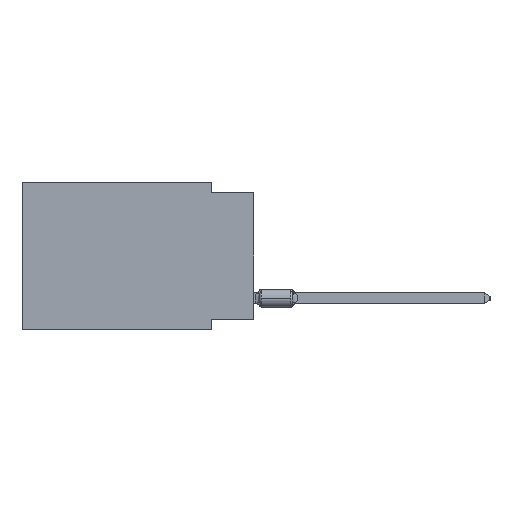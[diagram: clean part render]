
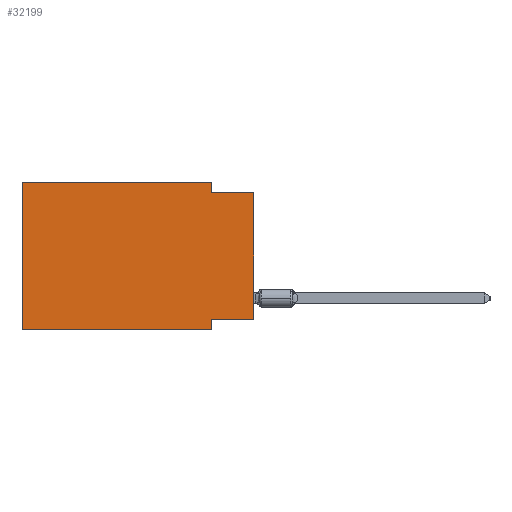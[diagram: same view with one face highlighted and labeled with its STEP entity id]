
A CAD part, left-side view. The second image highlights one B-rep face of the part: STEP entity #32199.
In plain terms, the highlighted planar face has unit normal (-1, 0, 0).
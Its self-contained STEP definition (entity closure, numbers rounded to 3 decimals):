
#111 = VERTEX_POINT ( 'NONE', #38459 ) ;
#2498 = VERTEX_POINT ( 'NONE', #49834 ) ;
#2507 = LINE ( 'NONE', #41799, #22081 ) ;
#3104 = VECTOR ( 'NONE', #41889, 1000. ) ;
#3886 = CARTESIAN_POINT ( 'NONE',  ( 0., 2.54, -8.89 ) ) ;
#4324 = VERTEX_POINT ( 'NONE', #9646 ) ;
#5627 = CARTESIAN_POINT ( 'NONE',  ( 0., 0., -8.255 ) ) ;
#5662 = LINE ( 'NONE', #8331, #18094 ) ;
#5913 = ORIENTED_EDGE ( 'NONE', *, *, #46895, .T. ) ;
#6121 = FACE_OUTER_BOUND ( 'NONE', #7224, .T. ) ;
#7224 = EDGE_LOOP ( 'NONE', ( #5913, #9223, #38173, #33896, #36323, #14181, #13645, #19008 ) ) ;
#7645 = VERTEX_POINT ( 'NONE', #42809 ) ;
#8331 = CARTESIAN_POINT ( 'NONE',  ( 0., 0., 0. ) ) ;
#8529 = CARTESIAN_POINT ( 'NONE',  ( 0., 13.97, 0. ) ) ;
#9223 = ORIENTED_EDGE ( 'NONE', *, *, #9245, .F. ) ;
#9245 = EDGE_CURVE ( 'NONE', #111, #46246, #42294, .T. ) ;
#9646 = CARTESIAN_POINT ( 'NONE',  ( 0., 2.54, -8.89 ) ) ;
#13481 = CARTESIAN_POINT ( 'NONE',  ( 0., 0., -8.255 ) ) ;
#13645 = ORIENTED_EDGE ( 'NONE', *, *, #26858, .F. ) ;
#14181 = ORIENTED_EDGE ( 'NONE', *, *, #25070, .T. ) ;
#14355 = VERTEX_POINT ( 'NONE', #46400 ) ;
#18094 = VECTOR ( 'NONE', #47621, 1000. ) ;
#19008 = ORIENTED_EDGE ( 'NONE', *, *, #35402, .F. ) ;
#20222 = VERTEX_POINT ( 'NONE', #45317 ) ;
#20427 = LINE ( 'NONE', #8529, #28915 ) ;
#22081 = VECTOR ( 'NONE', #25764, 1000. ) ;
#23148 = EDGE_CURVE ( 'NONE', #2498, #7645, #20427, .T. ) ;
#23711 = VERTEX_POINT ( 'NONE', #5627 ) ;
#23980 = VECTOR ( 'NONE', #44323, 1000. ) ;
#25070 = EDGE_CURVE ( 'NONE', #20222, #4324, #39927, .T. ) ;
#25526 = DIRECTION ( 'NONE',  ( 1., 0., 0. ) ) ;
#25648 = DIRECTION ( 'NONE',  ( 0., 1., 0. ) ) ;
#25764 = DIRECTION ( 'NONE',  ( 0., 0., -1. ) ) ;
#26736 = CARTESIAN_POINT ( 'NONE',  ( 0., 0., -0.635 ) ) ;
#26858 = EDGE_CURVE ( 'NONE', #14355, #4324, #26892, .T. ) ;
#26892 = LINE ( 'NONE', #3886, #45112 ) ;
#28286 = EDGE_CURVE ( 'NONE', #20222, #2498, #29974, .T. ) ;
#28424 = DIRECTION ( 'NONE',  ( 0., -1., 0. ) ) ;
#28915 = VECTOR ( 'NONE', #28424, 1000. ) ;
#29974 = LINE ( 'NONE', #45507, #3104 ) ;
#32199 = ADVANCED_FACE ( 'NONE', ( #6121 ), #37960, .F. ) ;
#33797 = CARTESIAN_POINT ( 'NONE',  ( 0., 0., -0.635 ) ) ;
#33896 = ORIENTED_EDGE ( 'NONE', *, *, #23148, .F. ) ;
#34510 = EDGE_CURVE ( 'NONE', #7645, #111, #2507, .T. ) ;
#35402 = EDGE_CURVE ( 'NONE', #23711, #14355, #48918, .T. ) ;
#36057 = CARTESIAN_POINT ( 'NONE',  ( 0., 13.97, -8.89 ) ) ;
#36323 = ORIENTED_EDGE ( 'NONE', *, *, #28286, .F. ) ;
#37687 = DIRECTION ( 'NONE',  ( 0., 0., -1. ) ) ;
#37960 = PLANE ( 'NONE',  #41874 ) ;
#38173 = ORIENTED_EDGE ( 'NONE', *, *, #34510, .F. ) ;
#38459 = CARTESIAN_POINT ( 'NONE',  ( 0., 2.54, -0.635 ) ) ;
#38662 = DIRECTION ( 'NONE',  ( 0., -1., 0. ) ) ;
#39587 = DIRECTION ( 'NONE',  ( 0., 0., -1. ) ) ;
#39927 = LINE ( 'NONE', #36057, #23980 ) ;
#41799 = CARTESIAN_POINT ( 'NONE',  ( 0., 2.54, 0. ) ) ;
#41874 = AXIS2_PLACEMENT_3D ( 'NONE', #49050, #25526, #37687 ) ;
#41889 = DIRECTION ( 'NONE',  ( 0., 0., 1. ) ) ;
#42294 = LINE ( 'NONE', #26736, #49245 ) ;
#42809 = CARTESIAN_POINT ( 'NONE',  ( 0., 2.54, 0. ) ) ;
#44323 = DIRECTION ( 'NONE',  ( 0., -1., 0. ) ) ;
#45112 = VECTOR ( 'NONE', #39587, 1000. ) ;
#45317 = CARTESIAN_POINT ( 'NONE',  ( 0., 13.97, -8.89 ) ) ;
#45507 = CARTESIAN_POINT ( 'NONE',  ( 0., 13.97, 0. ) ) ;
#46246 = VERTEX_POINT ( 'NONE', #33797 ) ;
#46400 = CARTESIAN_POINT ( 'NONE',  ( 0., 2.54, -8.255 ) ) ;
#46895 = EDGE_CURVE ( 'NONE', #23711, #46246, #5662, .T. ) ;
#47621 = DIRECTION ( 'NONE',  ( 0., 0., 1. ) ) ;
#48918 = LINE ( 'NONE', #13481, #49405 ) ;
#49050 = CARTESIAN_POINT ( 'NONE',  ( 0., 13.97, 0. ) ) ;
#49245 = VECTOR ( 'NONE', #38662, 1000. ) ;
#49405 = VECTOR ( 'NONE', #25648, 1000. ) ;
#49834 = CARTESIAN_POINT ( 'NONE',  ( 0., 13.97, 0. ) ) ;
